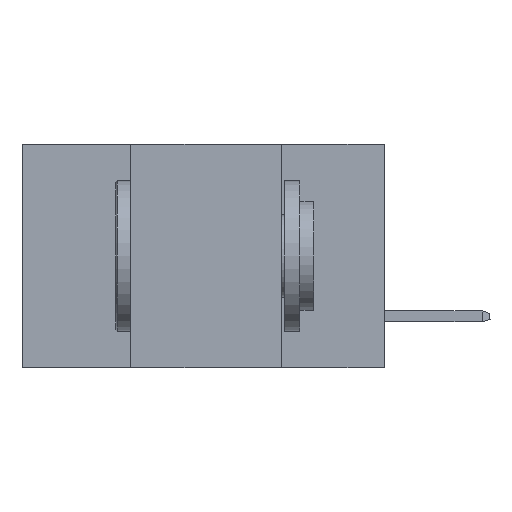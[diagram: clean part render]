
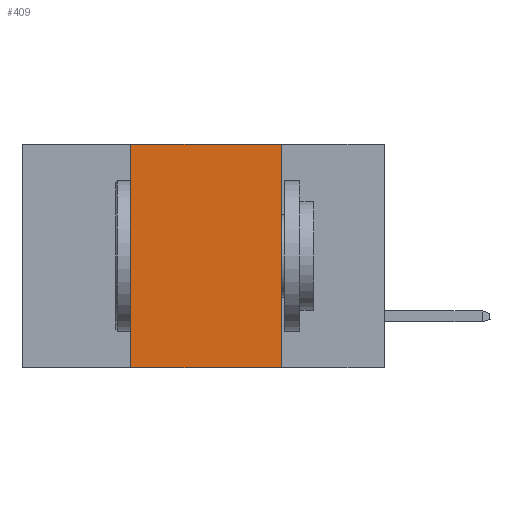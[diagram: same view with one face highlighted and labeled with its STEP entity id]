
A CAD part, left-side view. The second image highlights one B-rep face of the part: STEP entity #409.
In plain terms, the highlighted planar face has unit normal (-1, 0, 0).
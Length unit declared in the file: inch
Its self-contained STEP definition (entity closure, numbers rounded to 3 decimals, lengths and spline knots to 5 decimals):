
#409 = ADVANCED_FACE ( 'NONE', ( #10718 ), #20986, .F. ) ;
#819 = DIRECTION ( 'NONE',  ( 0., -1., 0. ) ) ;
#904 = VERTEX_POINT ( 'NONE', #5992 ) ;
#1402 = CARTESIAN_POINT ( 'NONE',  ( 0., 0.17, 0. ) ) ;
#1560 = CARTESIAN_POINT ( 'NONE',  ( 0., 0.42, 0. ) ) ;
#1955 = EDGE_CURVE ( 'NONE', #22272, #13485, #4769, .T. ) ;
#1978 = CARTESIAN_POINT ( 'NONE',  ( 0., 0.6, -0.37 ) ) ;
#3121 = EDGE_CURVE ( 'NONE', #13485, #904, #4431, .T. ) ;
#4431 = LINE ( 'NONE', #1402, #21881 ) ;
#4769 = LINE ( 'NONE', #13851, #17322 ) ;
#5992 = CARTESIAN_POINT ( 'NONE',  ( 0., 0.17, -0.37 ) ) ;
#6095 = DIRECTION ( 'NONE',  ( 1., 0., 0. ) ) ;
#6910 = VECTOR ( 'NONE', #18832, 39.37008 ) ;
#8131 = EDGE_CURVE ( 'NONE', #15651, #22272, #9602, .T. ) ;
#8166 = DIRECTION ( 'NONE',  ( 0., 0., -1. ) ) ;
#9602 = LINE ( 'NONE', #12828, #10180 ) ;
#10180 = VECTOR ( 'NONE', #23967, 39.37008 ) ;
#10718 = FACE_OUTER_BOUND ( 'NONE', #17219, .T. ) ;
#10898 = CARTESIAN_POINT ( 'NONE',  ( 0., 0.17, 0. ) ) ;
#11865 = EDGE_CURVE ( 'NONE', #15651, #904, #11887, .T. ) ;
#11887 = LINE ( 'NONE', #1978, #6910 ) ;
#12529 = ORIENTED_EDGE ( 'NONE', *, *, #1955, .F. ) ;
#12828 = CARTESIAN_POINT ( 'NONE',  ( 0., 0.42, 0. ) ) ;
#12959 = DIRECTION ( 'NONE',  ( 0., 0., -1. ) ) ;
#13485 = VERTEX_POINT ( 'NONE', #10898 ) ;
#13851 = CARTESIAN_POINT ( 'NONE',  ( 0., 0.6, 0. ) ) ;
#15455 = CARTESIAN_POINT ( 'NONE',  ( 0., 0.6, 0. ) ) ;
#15651 = VERTEX_POINT ( 'NONE', #19106 ) ;
#16265 = ORIENTED_EDGE ( 'NONE', *, *, #11865, .T. ) ;
#17219 = EDGE_LOOP ( 'NONE', ( #17685, #12529, #23245, #16265 ) ) ;
#17322 = VECTOR ( 'NONE', #819, 39.37008 ) ;
#17685 = ORIENTED_EDGE ( 'NONE', *, *, #3121, .F. ) ;
#18832 = DIRECTION ( 'NONE',  ( 0., -1., 0. ) ) ;
#19106 = CARTESIAN_POINT ( 'NONE',  ( 0., 0.42, -0.37 ) ) ;
#20986 = PLANE ( 'NONE',  #24106 ) ;
#21881 = VECTOR ( 'NONE', #12959, 39.37008 ) ;
#22272 = VERTEX_POINT ( 'NONE', #1560 ) ;
#23245 = ORIENTED_EDGE ( 'NONE', *, *, #8131, .F. ) ;
#23967 = DIRECTION ( 'NONE',  ( 0., 0., 1. ) ) ;
#24106 = AXIS2_PLACEMENT_3D ( 'NONE', #15455, #6095, #8166 ) ;
